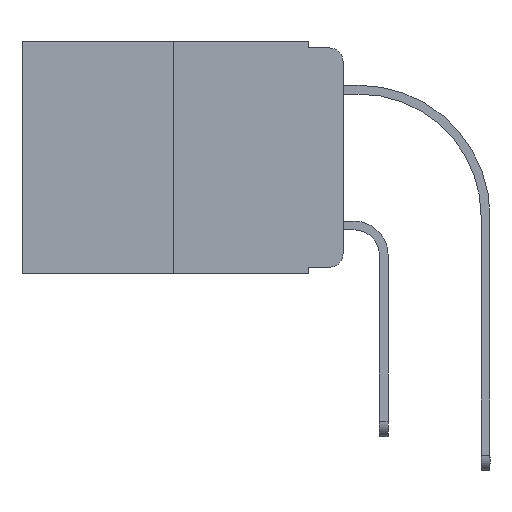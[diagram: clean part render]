
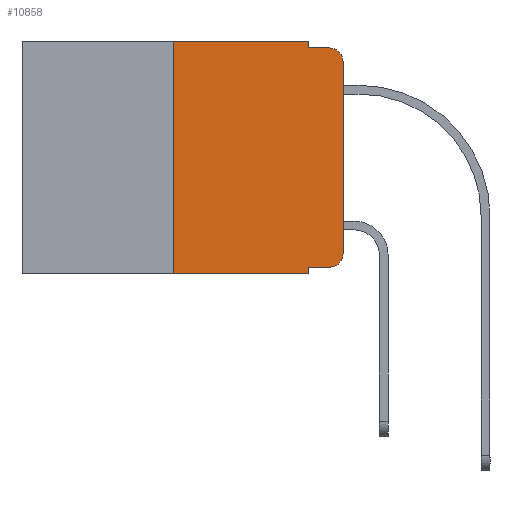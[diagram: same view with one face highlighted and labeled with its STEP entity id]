
A CAD part, left-side view. The second image highlights one B-rep face of the part: STEP entity #10858.
In plain terms, the highlighted planar face has unit normal (-1, 0, 0).
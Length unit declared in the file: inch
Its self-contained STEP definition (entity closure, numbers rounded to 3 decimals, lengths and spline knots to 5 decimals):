
#196 = CARTESIAN_POINT ( 'NONE',  ( 0., 0.051, -0.01 ) ) ;
#288 = CARTESIAN_POINT ( 'NONE',  ( 0., 0., -0.03 ) ) ;
#370 = VERTEX_POINT ( 'NONE', #288 ) ;
#385 = CARTESIAN_POINT ( 'NONE',  ( 0., 0.051, 0. ) ) ;
#488 = VECTOR ( 'NONE', #7759, 39.37008 ) ;
#558 = CARTESIAN_POINT ( 'NONE',  ( 0., 0.051, 0. ) ) ;
#592 = DIRECTION ( 'NONE',  ( 0., 0., 1. ) ) ;
#678 = AXIS2_PLACEMENT_3D ( 'NONE', #7570, #4656, #5507 ) ;
#682 = LINE ( 'NONE', #558, #1291 ) ;
#829 = CARTESIAN_POINT ( 'NONE',  ( 0., 0.25, 0. ) ) ;
#965 = ORIENTED_EDGE ( 'NONE', *, *, #6817, .T. ) ;
#992 = DIRECTION ( 'NONE',  ( 0., -1., 0. ) ) ;
#1119 = ORIENTED_EDGE ( 'NONE', *, *, #10033, .F. ) ;
#1291 = VECTOR ( 'NONE', #2322, 39.37008 ) ;
#1449 = CARTESIAN_POINT ( 'NONE',  ( 0., 0.473, 0. ) ) ;
#1623 = LINE ( 'NONE', #829, #9931 ) ;
#1997 = CARTESIAN_POINT ( 'NONE',  ( 0., 0.051, -0.333 ) ) ;
#2026 = VERTEX_POINT ( 'NONE', #9153 ) ;
#2110 = VERTEX_POINT ( 'NONE', #11223 ) ;
#2322 = DIRECTION ( 'NONE',  ( 0., 0., -1. ) ) ;
#2609 = DIRECTION ( 'NONE',  ( 0., -1., 0. ) ) ;
#2694 = CARTESIAN_POINT ( 'NONE',  ( 0., 0.051, -0.01 ) ) ;
#2721 = CARTESIAN_POINT ( 'NONE',  ( 0., 0., 0. ) ) ;
#2730 = DIRECTION ( 'NONE',  ( 0., -1., 0. ) ) ;
#2794 = VERTEX_POINT ( 'NONE', #4386 ) ;
#2837 = ORIENTED_EDGE ( 'NONE', *, *, #6856, .F. ) ;
#2848 = EDGE_CURVE ( 'NONE', #370, #5326, #9287, .T. ) ;
#3069 = EDGE_CURVE ( 'NONE', #4374, #7665, #4973, .T. ) ;
#3147 = CARTESIAN_POINT ( 'NONE',  ( 0., 0.02, -0.01 ) ) ;
#3440 = DIRECTION ( 'NONE',  ( 0., 0., 1. ) ) ;
#3465 = CARTESIAN_POINT ( 'NONE',  ( 0., 0.02, -0.03 ) ) ;
#3521 = ORIENTED_EDGE ( 'NONE', *, *, #2848, .T. ) ;
#3739 = ORIENTED_EDGE ( 'NONE', *, *, #8090, .F. ) ;
#3981 = AXIS2_PLACEMENT_3D ( 'NONE', #3465, #5353, #11849 ) ;
#4374 = VERTEX_POINT ( 'NONE', #1997 ) ;
#4386 = CARTESIAN_POINT ( 'NONE',  ( 0., 0., -0.313 ) ) ;
#4613 = CARTESIAN_POINT ( 'NONE',  ( 0., 0.051, 0. ) ) ;
#4656 = DIRECTION ( 'NONE',  ( -1., 0., 0. ) ) ;
#4686 = EDGE_CURVE ( 'NONE', #2794, #370, #5270, .T. ) ;
#4802 = EDGE_CURVE ( 'NONE', #7665, #2794, #9014, .T. ) ;
#4879 = VERTEX_POINT ( 'NONE', #385 ) ;
#4973 = LINE ( 'NONE', #5884, #488 ) ;
#5034 = VECTOR ( 'NONE', #992, 39.37008 ) ;
#5162 = VERTEX_POINT ( 'NONE', #5493 ) ;
#5270 = LINE ( 'NONE', #2721, #7649 ) ;
#5326 = VERTEX_POINT ( 'NONE', #3147 ) ;
#5339 = CARTESIAN_POINT ( 'NONE',  ( 0., 0.473, -0.343 ) ) ;
#5353 = DIRECTION ( 'NONE',  ( -1., 0., 0. ) ) ;
#5493 = CARTESIAN_POINT ( 'NONE',  ( 0., 0.051, -0.343 ) ) ;
#5507 = DIRECTION ( 'NONE',  ( 0., 0., -1. ) ) ;
#5610 = VECTOR ( 'NONE', #2730, 39.37008 ) ;
#5799 = VECTOR ( 'NONE', #2609, 39.37008 ) ;
#5884 = CARTESIAN_POINT ( 'NONE',  ( 0., 0.051, -0.333 ) ) ;
#5895 = EDGE_CURVE ( 'NONE', #9976, #5326, #11016, .T. ) ;
#6500 = LINE ( 'NONE', #4613, #10313 ) ;
#6623 = EDGE_LOOP ( 'NONE', ( #11214, #3521, #7408, #3739, #2837, #7909, #965, #1119, #11651, #10678 ) ) ;
#6817 = EDGE_CURVE ( 'NONE', #2026, #5162, #9157, .T. ) ;
#6856 = EDGE_CURVE ( 'NONE', #2110, #4879, #7158, .T. ) ;
#7158 = LINE ( 'NONE', #11046, #5610 ) ;
#7408 = ORIENTED_EDGE ( 'NONE', *, *, #5895, .F. ) ;
#7570 = CARTESIAN_POINT ( 'NONE',  ( 0., 0.02, -0.313 ) ) ;
#7649 = VECTOR ( 'NONE', #592, 39.37008 ) ;
#7665 = VERTEX_POINT ( 'NONE', #8269 ) ;
#7759 = DIRECTION ( 'NONE',  ( 0., -1., 0. ) ) ;
#7909 = ORIENTED_EDGE ( 'NONE', *, *, #8470, .F. ) ;
#8090 = EDGE_CURVE ( 'NONE', #4879, #9976, #6500, .T. ) ;
#8269 = CARTESIAN_POINT ( 'NONE',  ( 0., 0.02, -0.333 ) ) ;
#8315 = DIRECTION ( 'NONE',  ( 0., 0., -1. ) ) ;
#8470 = EDGE_CURVE ( 'NONE', #2026, #2110, #1623, .T. ) ;
#9014 = CIRCLE ( 'NONE', #678, 0.02 ) ;
#9153 = CARTESIAN_POINT ( 'NONE',  ( 0., 0.25, -0.343 ) ) ;
#9157 = LINE ( 'NONE', #5339, #5799 ) ;
#9287 = CIRCLE ( 'NONE', #3981, 0.02 ) ;
#9610 = AXIS2_PLACEMENT_3D ( 'NONE', #1449, #9700, #11714 ) ;
#9700 = DIRECTION ( 'NONE',  ( 1., 0., 0. ) ) ;
#9767 = FACE_OUTER_BOUND ( 'NONE', #6623, .T. ) ;
#9827 = PLANE ( 'NONE',  #9610 ) ;
#9931 = VECTOR ( 'NONE', #3440, 39.37008 ) ;
#9976 = VERTEX_POINT ( 'NONE', #196 ) ;
#10033 = EDGE_CURVE ( 'NONE', #4374, #5162, #682, .T. ) ;
#10313 = VECTOR ( 'NONE', #8315, 39.37008 ) ;
#10678 = ORIENTED_EDGE ( 'NONE', *, *, #4802, .T. ) ;
#10858 = ADVANCED_FACE ( 'NONE', ( #9767 ), #9827, .F. ) ;
#11016 = LINE ( 'NONE', #2694, #5034 ) ;
#11046 = CARTESIAN_POINT ( 'NONE',  ( 0., 0.473, 0. ) ) ;
#11214 = ORIENTED_EDGE ( 'NONE', *, *, #4686, .T. ) ;
#11223 = CARTESIAN_POINT ( 'NONE',  ( 0., 0.25, 0. ) ) ;
#11651 = ORIENTED_EDGE ( 'NONE', *, *, #3069, .T. ) ;
#11714 = DIRECTION ( 'NONE',  ( 0., 0., -1. ) ) ;
#11849 = DIRECTION ( 'NONE',  ( 0., 0., -1. ) ) ;
